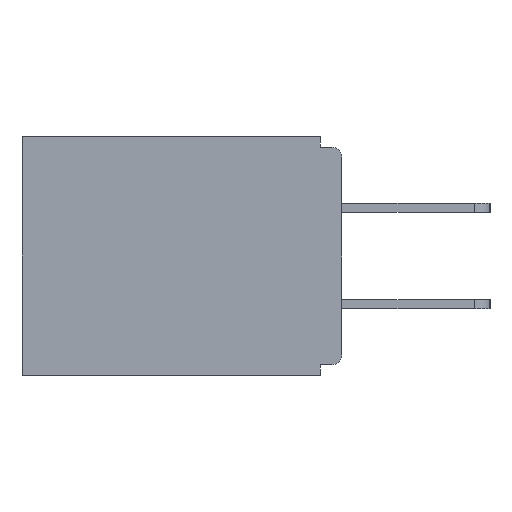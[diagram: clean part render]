
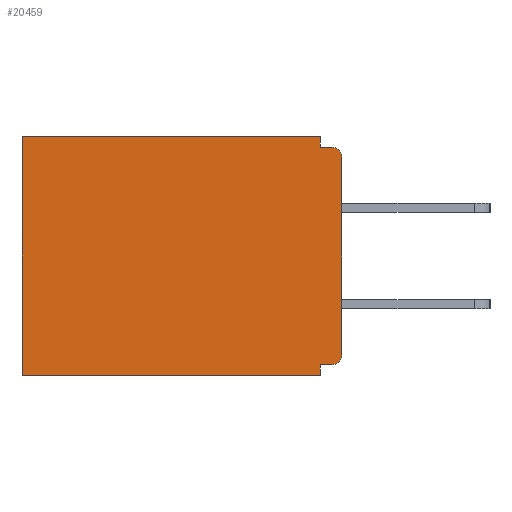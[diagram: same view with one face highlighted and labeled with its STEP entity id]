
A CAD part, left-side view. The second image highlights one B-rep face of the part: STEP entity #20459.
In plain terms, the highlighted planar face has unit normal (-1, 0, 0).
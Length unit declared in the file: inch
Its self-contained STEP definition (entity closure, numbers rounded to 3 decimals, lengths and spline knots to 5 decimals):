
#114 = CARTESIAN_POINT ( 'NONE',  ( 0.298, 0., -0.343 ) ) ;
#677 = VECTOR ( 'NONE', #12669, 39.37008 ) ;
#678 = VECTOR ( 'NONE', #2105, 39.37008 ) ;
#1431 = CARTESIAN_POINT ( 'NONE',  ( 0.298, 0.46, 0. ) ) ;
#1588 = LINE ( 'NONE', #6632, #15749 ) ;
#2105 = DIRECTION ( 'NONE',  ( 0., 0., -1. ) ) ;
#2441 = VERTEX_POINT ( 'NONE', #18099 ) ;
#2508 = CARTESIAN_POINT ( 'NONE',  ( 0.298, 0.015, -0.015 ) ) ;
#2689 = ORIENTED_EDGE ( 'NONE', *, *, #18882, .F. ) ;
#2788 = DIRECTION ( 'NONE',  ( -1., 0., 0. ) ) ;
#3451 = CARTESIAN_POINT ( 'NONE',  ( 0.298, 0.46, -0.343 ) ) ;
#3454 = ORIENTED_EDGE ( 'NONE', *, *, #17852, .T. ) ;
#3470 = DIRECTION ( 'NONE',  ( 0., 0., -1. ) ) ;
#3564 = ORIENTED_EDGE ( 'NONE', *, *, #7532, .F. ) ;
#3608 = ORIENTED_EDGE ( 'NONE', *, *, #15543, .T. ) ;
#3746 = CARTESIAN_POINT ( 'NONE',  ( 0.298, 0.031, -0.328 ) ) ;
#3974 = ORIENTED_EDGE ( 'NONE', *, *, #16615, .F. ) ;
#4232 = EDGE_CURVE ( 'NONE', #13610, #20289, #7918, .T. ) ;
#4811 = VERTEX_POINT ( 'NONE', #3451 ) ;
#5311 = LINE ( 'NONE', #6938, #677 ) ;
#5619 = DIRECTION ( 'NONE',  ( 0., 0., -1. ) ) ;
#5962 = FACE_OUTER_BOUND ( 'NONE', #20938, .T. ) ;
#6227 = VERTEX_POINT ( 'NONE', #8870 ) ;
#6483 = EDGE_CURVE ( 'NONE', #13948, #12042, #8071, .T. ) ;
#6630 = VECTOR ( 'NONE', #9427, 39.37008 ) ;
#6632 = CARTESIAN_POINT ( 'NONE',  ( 0.298, 0., -0.015 ) ) ;
#6938 = CARTESIAN_POINT ( 'NONE',  ( 0.298, 0., -0.328 ) ) ;
#7058 = VECTOR ( 'NONE', #20654, 39.37008 ) ;
#7532 = EDGE_CURVE ( 'NONE', #2441, #9215, #10182, .T. ) ;
#7861 = ORIENTED_EDGE ( 'NONE', *, *, #8774, .T. ) ;
#7918 = LINE ( 'NONE', #11665, #678 ) ;
#7936 = CARTESIAN_POINT ( 'NONE',  ( 0.298, 0., 0. ) ) ;
#8071 = LINE ( 'NONE', #18737, #6630 ) ;
#8108 = VECTOR ( 'NONE', #14277, 39.37008 ) ;
#8774 = EDGE_CURVE ( 'NONE', #12042, #4811, #23455, .T. ) ;
#8870 = CARTESIAN_POINT ( 'NONE',  ( 0.298, 0.031, -0.015 ) ) ;
#9105 = CARTESIAN_POINT ( 'NONE',  ( 0.298, 0.031, -0.343 ) ) ;
#9215 = VERTEX_POINT ( 'NONE', #9624 ) ;
#9427 = DIRECTION ( 'NONE',  ( 0., 1., 0. ) ) ;
#9559 = CARTESIAN_POINT ( 'NONE',  ( 0.298, 0.015, -0.313 ) ) ;
#9624 = CARTESIAN_POINT ( 'NONE',  ( 0.298, 0., -0.313 ) ) ;
#9827 = VERTEX_POINT ( 'NONE', #18039 ) ;
#10182 = LINE ( 'NONE', #22369, #17691 ) ;
#10629 = CARTESIAN_POINT ( 'NONE',  ( 0.298, 0.46, 0. ) ) ;
#11240 = CARTESIAN_POINT ( 'NONE',  ( 0.298, 0.031, 0. ) ) ;
#11552 = DIRECTION ( 'NONE',  ( 0., 0., -1. ) ) ;
#11665 = CARTESIAN_POINT ( 'NONE',  ( 0.298, 0.031, -0.343 ) ) ;
#12042 = VERTEX_POINT ( 'NONE', #10629 ) ;
#12374 = CARTESIAN_POINT ( 'NONE',  ( 0.298, 0.031, -0.343 ) ) ;
#12669 = DIRECTION ( 'NONE',  ( 0., 1., 0. ) ) ;
#12716 = VERTEX_POINT ( 'NONE', #2508 ) ;
#12991 = LINE ( 'NONE', #9105, #13272 ) ;
#13272 = VECTOR ( 'NONE', #3470, 39.37008 ) ;
#13320 = ORIENTED_EDGE ( 'NONE', *, *, #4232, .F. ) ;
#13461 = ORIENTED_EDGE ( 'NONE', *, *, #21197, .F. ) ;
#13610 = VERTEX_POINT ( 'NONE', #3746 ) ;
#13741 = DIRECTION ( 'NONE',  ( 0., -1., 0. ) ) ;
#13948 = VERTEX_POINT ( 'NONE', #11240 ) ;
#14216 = ORIENTED_EDGE ( 'NONE', *, *, #16117, .F. ) ;
#14277 = DIRECTION ( 'NONE',  ( 0., 0., -1. ) ) ;
#15542 = AXIS2_PLACEMENT_3D ( 'NONE', #9559, #18953, #19111 ) ;
#15543 = EDGE_CURVE ( 'NONE', #2441, #12716, #20424, .T. ) ;
#15749 = VECTOR ( 'NONE', #13741, 39.37008 ) ;
#15780 = CARTESIAN_POINT ( 'NONE',  ( 0.298, 0.015, -0.03 ) ) ;
#15825 = AXIS2_PLACEMENT_3D ( 'NONE', #15780, #2788, #19515 ) ;
#16117 = EDGE_CURVE ( 'NONE', #6227, #12716, #1588, .T. ) ;
#16615 = EDGE_CURVE ( 'NONE', #9827, #13610, #5311, .T. ) ;
#17073 = ORIENTED_EDGE ( 'NONE', *, *, #6483, .T. ) ;
#17282 = PLANE ( 'NONE',  #19936 ) ;
#17691 = VECTOR ( 'NONE', #5619, 39.37008 ) ;
#17852 = EDGE_CURVE ( 'NONE', #9827, #9215, #18815, .T. ) ;
#18031 = LINE ( 'NONE', #114, #7058 ) ;
#18039 = CARTESIAN_POINT ( 'NONE',  ( 0.298, 0.015, -0.328 ) ) ;
#18099 = CARTESIAN_POINT ( 'NONE',  ( 0.298, 0., -0.03 ) ) ;
#18737 = CARTESIAN_POINT ( 'NONE',  ( 0.298, 0., 0. ) ) ;
#18815 = CIRCLE ( 'NONE', #15542, 0.015 ) ;
#18882 = EDGE_CURVE ( 'NONE', #13948, #6227, #12991, .T. ) ;
#18953 = DIRECTION ( 'NONE',  ( -1., 0., 0. ) ) ;
#19111 = DIRECTION ( 'NONE',  ( 0., 0., -1. ) ) ;
#19515 = DIRECTION ( 'NONE',  ( 0., 0., -1. ) ) ;
#19936 = AXIS2_PLACEMENT_3D ( 'NONE', #7936, #21050, #11552 ) ;
#20289 = VERTEX_POINT ( 'NONE', #12374 ) ;
#20424 = CIRCLE ( 'NONE', #15825, 0.015 ) ;
#20459 = ADVANCED_FACE ( 'NONE', ( #5962 ), #17282, .F. ) ;
#20654 = DIRECTION ( 'NONE',  ( 0., 1., 0. ) ) ;
#20938 = EDGE_LOOP ( 'NONE', ( #3608, #14216, #2689, #17073, #7861, #13461, #13320, #3974, #3454, #3564 ) ) ;
#21050 = DIRECTION ( 'NONE',  ( 1., 0., 0. ) ) ;
#21197 = EDGE_CURVE ( 'NONE', #20289, #4811, #18031, .T. ) ;
#22369 = CARTESIAN_POINT ( 'NONE',  ( 0.298, 0., 0. ) ) ;
#23455 = LINE ( 'NONE', #1431, #8108 ) ;
